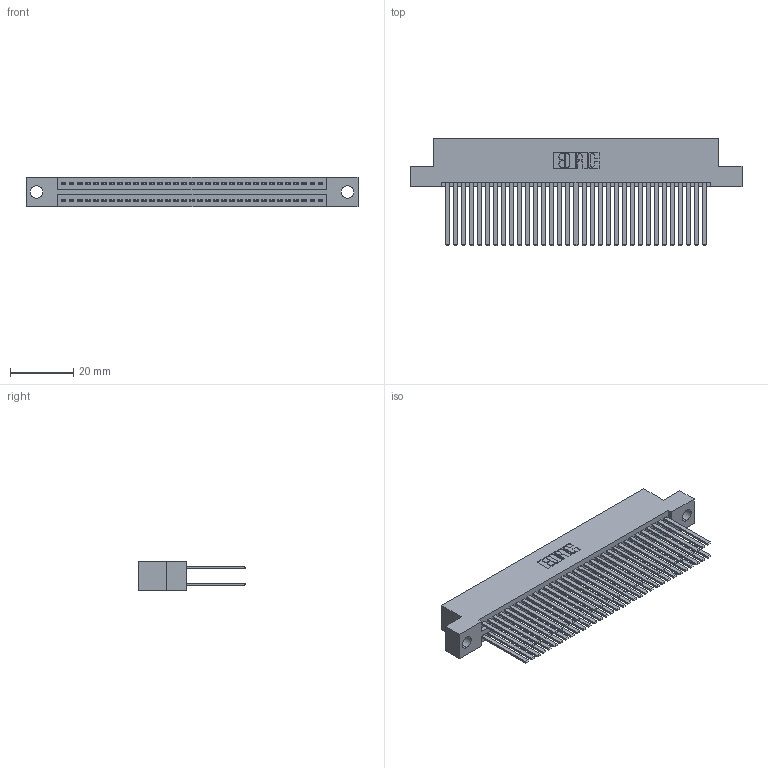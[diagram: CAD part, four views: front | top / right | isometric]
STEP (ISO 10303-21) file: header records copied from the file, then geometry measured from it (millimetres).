
FILE_DESCRIPTION (( 'STEP AP203' ), '1' );
FILE_NAME ('395-066-544-204.STEP', '2021-06-17T03:33:04', ( '' ), ( '' ), 'SwSTEP 2.0', 'SolidWorks 2020', '' );
FILE_SCHEMA (( 'CONFIG_CONTROL_DESIGN' ));
Length unit declared in the file: inch
Products named in the file (3): 345-292-001_345-293-144; 345 Part_Flush Mounting Lugs - 0.156 Dia-TI; 395-066-544-204
Assembly tree (67 placements, depth 2):
  395-066-544-204
    345 Part_Flush Mounting Lugs - 0.156 Dia-TI
    345-292-001_345-293-144  x66
Bounding box: 105.03 x 33.96 x 9.4 mm (x, y, z)
Volume: 10938.3 mm3; surface area: 18557.6 mm2
Topology: 67 solids, 67 shells, 3044 faces, 9023 edges, 5926 vertices
Faces by surface type: plane 2008, cylinder 1036
Entity records: 27339 total; most frequent: CARTESIAN_POINT 4594, ORIENTED_EDGE 4526, DIRECTION 4059, EDGE_CURVE 2263, VECTOR 2003, LINE 2003, VERTEX_POINT 1506, AXIS2_PLACEMENT_3D 1028
